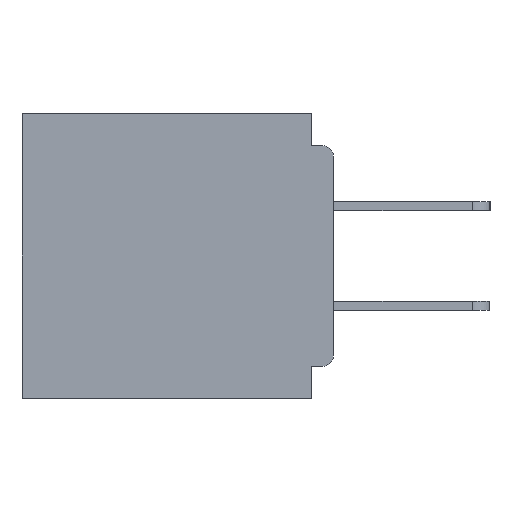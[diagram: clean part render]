
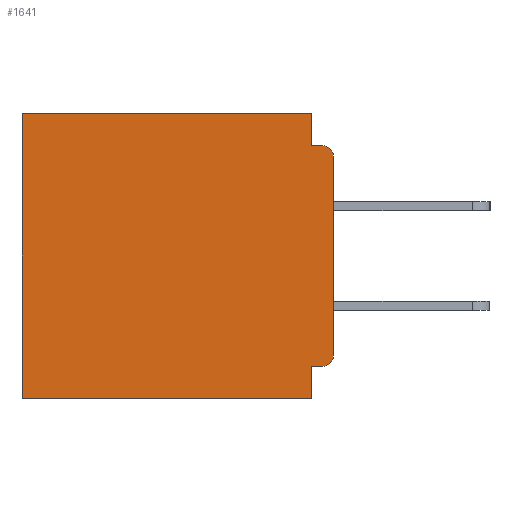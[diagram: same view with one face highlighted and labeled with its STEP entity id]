
A CAD part, left-side view. The second image highlights one B-rep face of the part: STEP entity #1641.
In plain terms, the highlighted planar face has unit normal (-1, 0, 0).
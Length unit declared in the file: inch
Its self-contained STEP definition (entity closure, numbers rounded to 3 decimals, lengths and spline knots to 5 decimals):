
#219 = DIRECTION ( 'NONE',  ( 0., 0., -1. ) ) ;
#594 = VECTOR ( 'NONE', #16314, 39.37008 ) ;
#620 = CARTESIAN_POINT ( 'NONE',  ( 0.3, 0., -0.045 ) ) ;
#1034 = EDGE_CURVE ( 'NONE', #28946, #32463, #14664, .T. ) ;
#1259 = FACE_OUTER_BOUND ( 'NONE', #10118, .T. ) ;
#1641 = ADVANCED_FACE ( 'NONE', ( #1259 ), #16196, .F. ) ;
#3154 = VERTEX_POINT ( 'NONE', #5924 ) ;
#3182 = CARTESIAN_POINT ( 'NONE',  ( 0.3, 0., -0.4 ) ) ;
#3494 = CARTESIAN_POINT ( 'NONE',  ( 0.3, 0., -0.06 ) ) ;
#3529 = VECTOR ( 'NONE', #23616, 39.37008 ) ;
#3532 = VECTOR ( 'NONE', #25511, 39.37008 ) ;
#4391 = LINE ( 'NONE', #29833, #13131 ) ;
#4700 = ORIENTED_EDGE ( 'NONE', *, *, #30113, .F. ) ;
#5114 = CARTESIAN_POINT ( 'NONE',  ( 0.3, 0.031, 0. ) ) ;
#5754 = LINE ( 'NONE', #620, #35693 ) ;
#5924 = CARTESIAN_POINT ( 'NONE',  ( 0.3, 0.031, -0.045 ) ) ;
#6787 = CARTESIAN_POINT ( 'NONE',  ( 0.3, 0.031, -0.355 ) ) ;
#6878 = VECTOR ( 'NONE', #7104, 39.37008 ) ;
#7104 = DIRECTION ( 'NONE',  ( 0., 0., -1. ) ) ;
#7247 = CARTESIAN_POINT ( 'NONE',  ( 0.3, 0., -0.4 ) ) ;
#7310 = CARTESIAN_POINT ( 'NONE',  ( 0.3, 0.437, -0.4 ) ) ;
#7380 = VERTEX_POINT ( 'NONE', #33473 ) ;
#8440 = LINE ( 'NONE', #18984, #23948 ) ;
#9154 = EDGE_CURVE ( 'NONE', #7380, #28946, #8440, .T. ) ;
#9407 = LINE ( 'NONE', #24930, #594 ) ;
#10002 = CARTESIAN_POINT ( 'NONE',  ( 0.3, 0.437, -0.4 ) ) ;
#10118 = EDGE_LOOP ( 'NONE', ( #19312, #30277, #12471, #34285, #11486, #14388, #31549, #35879, #4700, #17000 ) ) ;
#11138 = VECTOR ( 'NONE', #29298, 39.37008 ) ;
#11486 = ORIENTED_EDGE ( 'NONE', *, *, #9154, .T. ) ;
#11969 = DIRECTION ( 'NONE',  ( -1., 0., 0. ) ) ;
#12015 = EDGE_CURVE ( 'NONE', #29871, #24220, #17361, .T. ) ;
#12035 = AXIS2_PLACEMENT_3D ( 'NONE', #35095, #17844, #219 ) ;
#12471 = ORIENTED_EDGE ( 'NONE', *, *, #18487, .F. ) ;
#12480 = DIRECTION ( 'NONE',  ( 0., 0., -1. ) ) ;
#12495 = DIRECTION ( 'NONE',  ( 0., -1., 0. ) ) ;
#12657 = CARTESIAN_POINT ( 'NONE',  ( 0.3, 0.015, -0.355 ) ) ;
#13131 = VECTOR ( 'NONE', #12480, 39.37008 ) ;
#13190 = CARTESIAN_POINT ( 'NONE',  ( 0.3, 0.437, 0. ) ) ;
#13759 = AXIS2_PLACEMENT_3D ( 'NONE', #29329, #11969, #32222 ) ;
#14388 = ORIENTED_EDGE ( 'NONE', *, *, #1034, .T. ) ;
#14460 = EDGE_CURVE ( 'NONE', #16397, #20238, #27518, .T. ) ;
#14664 = LINE ( 'NONE', #7310, #6878 ) ;
#16196 = PLANE ( 'NONE',  #20049 ) ;
#16314 = DIRECTION ( 'NONE',  ( 0., 1., 0. ) ) ;
#16397 = VERTEX_POINT ( 'NONE', #6787 ) ;
#17000 = ORIENTED_EDGE ( 'NONE', *, *, #37019, .T. ) ;
#17361 = CIRCLE ( 'NONE', #13759, 0.015 ) ;
#17844 = DIRECTION ( 'NONE',  ( -1., 0., 0. ) ) ;
#18487 = EDGE_CURVE ( 'NONE', #3154, #24220, #5754, .T. ) ;
#18844 = CARTESIAN_POINT ( 'NONE',  ( 0.3, 0.015, -0.045 ) ) ;
#18984 = CARTESIAN_POINT ( 'NONE',  ( 0.3, 0., 0. ) ) ;
#19312 = ORIENTED_EDGE ( 'NONE', *, *, #35314, .F. ) ;
#20049 = AXIS2_PLACEMENT_3D ( 'NONE', #7247, #22630, #25635 ) ;
#20238 = VERTEX_POINT ( 'NONE', #32488 ) ;
#22630 = DIRECTION ( 'NONE',  ( 1., 0., 0. ) ) ;
#23616 = DIRECTION ( 'NONE',  ( 0., 1., 0. ) ) ;
#23948 = VECTOR ( 'NONE', #27717, 39.37008 ) ;
#24220 = VERTEX_POINT ( 'NONE', #18844 ) ;
#24930 = CARTESIAN_POINT ( 'NONE',  ( 0.3, 0., -0.355 ) ) ;
#25511 = DIRECTION ( 'NONE',  ( 0., 0., -1. ) ) ;
#25635 = DIRECTION ( 'NONE',  ( 0., 0., -1. ) ) ;
#25905 = LINE ( 'NONE', #5114, #3532 ) ;
#27518 = LINE ( 'NONE', #29175, #11138 ) ;
#27717 = DIRECTION ( 'NONE',  ( 0., 1., 0. ) ) ;
#28028 = CIRCLE ( 'NONE', #12035, 0.015 ) ;
#28685 = EDGE_CURVE ( 'NONE', #20238, #32463, #33524, .T. ) ;
#28946 = VERTEX_POINT ( 'NONE', #13190 ) ;
#29175 = CARTESIAN_POINT ( 'NONE',  ( 0.3, 0.031, -0.4 ) ) ;
#29298 = DIRECTION ( 'NONE',  ( 0., 0., -1. ) ) ;
#29329 = CARTESIAN_POINT ( 'NONE',  ( 0.3, 0.015, -0.06 ) ) ;
#29336 = VERTEX_POINT ( 'NONE', #12657 ) ;
#29833 = CARTESIAN_POINT ( 'NONE',  ( 0.3, 0., -0.4 ) ) ;
#29871 = VERTEX_POINT ( 'NONE', #3494 ) ;
#30113 = EDGE_CURVE ( 'NONE', #29336, #16397, #9407, .T. ) ;
#30277 = ORIENTED_EDGE ( 'NONE', *, *, #12015, .T. ) ;
#31549 = ORIENTED_EDGE ( 'NONE', *, *, #28685, .F. ) ;
#31959 = CARTESIAN_POINT ( 'NONE',  ( 0.3, 0., -0.34 ) ) ;
#32186 = VERTEX_POINT ( 'NONE', #31959 ) ;
#32222 = DIRECTION ( 'NONE',  ( 0., 0., -1. ) ) ;
#32463 = VERTEX_POINT ( 'NONE', #10002 ) ;
#32488 = CARTESIAN_POINT ( 'NONE',  ( 0.3, 0.031, -0.4 ) ) ;
#33473 = CARTESIAN_POINT ( 'NONE',  ( 0.3, 0.031, 0. ) ) ;
#33524 = LINE ( 'NONE', #3182, #3529 ) ;
#34285 = ORIENTED_EDGE ( 'NONE', *, *, #34478, .F. ) ;
#34478 = EDGE_CURVE ( 'NONE', #7380, #3154, #25905, .T. ) ;
#35095 = CARTESIAN_POINT ( 'NONE',  ( 0.3, 0.015, -0.34 ) ) ;
#35314 = EDGE_CURVE ( 'NONE', #29871, #32186, #4391, .T. ) ;
#35693 = VECTOR ( 'NONE', #12495, 39.37008 ) ;
#35879 = ORIENTED_EDGE ( 'NONE', *, *, #14460, .F. ) ;
#37019 = EDGE_CURVE ( 'NONE', #29336, #32186, #28028, .T. ) ;
